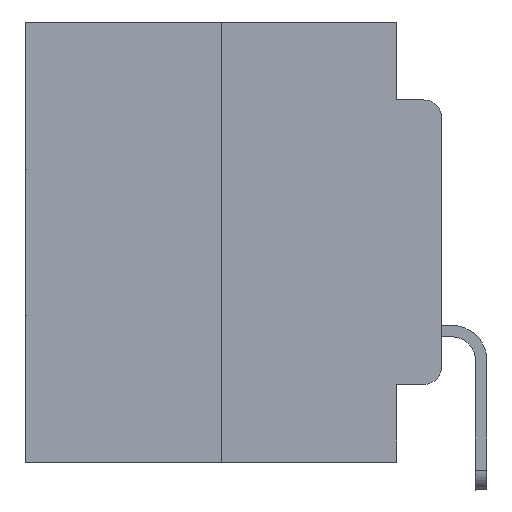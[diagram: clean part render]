
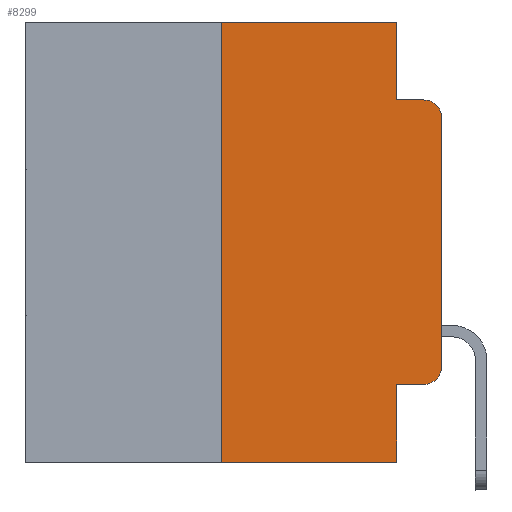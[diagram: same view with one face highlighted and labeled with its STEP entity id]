
A CAD part, left-side view. The second image highlights one B-rep face of the part: STEP entity #8299.
In plain terms, the highlighted planar face has unit normal (-1, 0, 0).
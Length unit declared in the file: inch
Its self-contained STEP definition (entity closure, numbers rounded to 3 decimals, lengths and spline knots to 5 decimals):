
#231 = EDGE_CURVE ( 'NONE', #22024, #13875, #4249, .T. ) ;
#243 = EDGE_CURVE ( 'NONE', #16934, #6753, #7136, .T. ) ;
#451 = CARTESIAN_POINT ( 'NONE',  ( 0., 0.051, 0. ) ) ;
#801 = ORIENTED_EDGE ( 'NONE', *, *, #7819, .T. ) ;
#1180 = AXIS2_PLACEMENT_3D ( 'NONE', #3368, #20275, #26350 ) ;
#1366 = EDGE_CURVE ( 'NONE', #1755, #2538, #14236, .T. ) ;
#1501 = EDGE_LOOP ( 'NONE', ( #801, #6724, #10126, #22751, #17772, #27119, #16622, #11106, #7341, #23350 ) ) ;
#1755 = VERTEX_POINT ( 'NONE', #24566 ) ;
#1921 = VERTEX_POINT ( 'NONE', #24707 ) ;
#2258 = LINE ( 'NONE', #17057, #8096 ) ;
#2538 = VERTEX_POINT ( 'NONE', #17056 ) ;
#3125 = CARTESIAN_POINT ( 'NONE',  ( 0., 0.02, -0.0885 ) ) ;
#3368 = CARTESIAN_POINT ( 'NONE',  ( 0., 0.473, 0. ) ) ;
#3680 = CARTESIAN_POINT ( 'NONE',  ( 0., 0.051, -0.4115 ) ) ;
#4249 = LINE ( 'NONE', #14787, #23830 ) ;
#4804 = LINE ( 'NONE', #21695, #24120 ) ;
#5696 = EDGE_CURVE ( 'NONE', #18847, #15049, #24532, .T. ) ;
#5939 = DIRECTION ( 'NONE',  ( -1., 0., 0. ) ) ;
#6724 = ORIENTED_EDGE ( 'NONE', *, *, #243, .T. ) ;
#6753 = VERTEX_POINT ( 'NONE', #3125 ) ;
#7136 = CIRCLE ( 'NONE', #12796, 0.02 ) ;
#7341 = ORIENTED_EDGE ( 'NONE', *, *, #8076, .T. ) ;
#7819 = EDGE_CURVE ( 'NONE', #15049, #16934, #9240, .T. ) ;
#7847 = EDGE_CURVE ( 'NONE', #1921, #22024, #4804, .T. ) ;
#7878 = CARTESIAN_POINT ( 'NONE',  ( 0., 0.02, -0.3915 ) ) ;
#7927 = CARTESIAN_POINT ( 'NONE',  ( 0., 0., -0.1085 ) ) ;
#8076 = EDGE_CURVE ( 'NONE', #1755, #18847, #10615, .T. ) ;
#8096 = VECTOR ( 'NONE', #25489, 39.37008 ) ;
#8299 = ADVANCED_FACE ( 'NONE', ( #9482 ), #19866, .F. ) ;
#8949 = EDGE_CURVE ( 'NONE', #13875, #24169, #19257, .T. ) ;
#9240 = LINE ( 'NONE', #15200, #13538 ) ;
#9482 = FACE_OUTER_BOUND ( 'NONE', #1501, .T. ) ;
#9534 = CARTESIAN_POINT ( 'NONE',  ( 0., 0.051, 0. ) ) ;
#10126 = ORIENTED_EDGE ( 'NONE', *, *, #25002, .F. ) ;
#10421 = AXIS2_PLACEMENT_3D ( 'NONE', #7878, #5939, #20496 ) ;
#10615 = LINE ( 'NONE', #3680, #26804 ) ;
#11106 = ORIENTED_EDGE ( 'NONE', *, *, #1366, .F. ) ;
#11527 = CARTESIAN_POINT ( 'NONE',  ( 0., 0.051, -0.0885 ) ) ;
#11593 = CARTESIAN_POINT ( 'NONE',  ( 0., 0.051, -0.0885 ) ) ;
#11717 = DIRECTION ( 'NONE',  ( 0., 0., 1. ) ) ;
#11862 = LINE ( 'NONE', #11593, #21523 ) ;
#12420 = DIRECTION ( 'NONE',  ( 0., -1., 0. ) ) ;
#12516 = CARTESIAN_POINT ( 'NONE',  ( 0., 0., -0.3915 ) ) ;
#12796 = AXIS2_PLACEMENT_3D ( 'NONE', #24731, #27213, #26945 ) ;
#13538 = VECTOR ( 'NONE', #15337, 39.37008 ) ;
#13875 = VERTEX_POINT ( 'NONE', #17110 ) ;
#14217 = DIRECTION ( 'NONE',  ( 0., -1., 0. ) ) ;
#14236 = LINE ( 'NONE', #9534, #20130 ) ;
#14787 = CARTESIAN_POINT ( 'NONE',  ( 0., 0.473, 0. ) ) ;
#15049 = VERTEX_POINT ( 'NONE', #12516 ) ;
#15200 = CARTESIAN_POINT ( 'NONE',  ( 0., 0., 0. ) ) ;
#15337 = DIRECTION ( 'NONE',  ( 0., 0., 1. ) ) ;
#16622 = ORIENTED_EDGE ( 'NONE', *, *, #19608, .T. ) ;
#16682 = VECTOR ( 'NONE', #25470, 39.37008 ) ;
#16703 = CARTESIAN_POINT ( 'NONE',  ( 0., 0.02, -0.4115 ) ) ;
#16934 = VERTEX_POINT ( 'NONE', #7927 ) ;
#17056 = CARTESIAN_POINT ( 'NONE',  ( 0., 0.051, -0.5 ) ) ;
#17057 = CARTESIAN_POINT ( 'NONE',  ( 0., 0.473, -0.5 ) ) ;
#17110 = CARTESIAN_POINT ( 'NONE',  ( 0., 0.051, 0. ) ) ;
#17772 = ORIENTED_EDGE ( 'NONE', *, *, #231, .F. ) ;
#18847 = VERTEX_POINT ( 'NONE', #16703 ) ;
#19257 = LINE ( 'NONE', #451, #16682 ) ;
#19608 = EDGE_CURVE ( 'NONE', #1921, #2538, #2258, .T. ) ;
#19866 = PLANE ( 'NONE',  #1180 ) ;
#20047 = DIRECTION ( 'NONE',  ( 0., -1., 0. ) ) ;
#20130 = VECTOR ( 'NONE', #26678, 39.37008 ) ;
#20275 = DIRECTION ( 'NONE',  ( 1., 0., 0. ) ) ;
#20496 = DIRECTION ( 'NONE',  ( 0., 0., -1. ) ) ;
#21523 = VECTOR ( 'NONE', #20047, 39.37008 ) ;
#21695 = CARTESIAN_POINT ( 'NONE',  ( 0., 0.25, 0. ) ) ;
#22024 = VERTEX_POINT ( 'NONE', #25775 ) ;
#22751 = ORIENTED_EDGE ( 'NONE', *, *, #8949, .F. ) ;
#23350 = ORIENTED_EDGE ( 'NONE', *, *, #5696, .T. ) ;
#23830 = VECTOR ( 'NONE', #12420, 39.37008 ) ;
#24120 = VECTOR ( 'NONE', #11717, 39.37008 ) ;
#24169 = VERTEX_POINT ( 'NONE', #11527 ) ;
#24532 = CIRCLE ( 'NONE', #10421, 0.02 ) ;
#24566 = CARTESIAN_POINT ( 'NONE',  ( 0., 0.051, -0.4115 ) ) ;
#24707 = CARTESIAN_POINT ( 'NONE',  ( 0., 0.25, -0.5 ) ) ;
#24731 = CARTESIAN_POINT ( 'NONE',  ( 0., 0.02, -0.1085 ) ) ;
#25002 = EDGE_CURVE ( 'NONE', #24169, #6753, #11862, .T. ) ;
#25470 = DIRECTION ( 'NONE',  ( 0., 0., -1. ) ) ;
#25489 = DIRECTION ( 'NONE',  ( 0., -1., 0. ) ) ;
#25775 = CARTESIAN_POINT ( 'NONE',  ( 0., 0.25, 0. ) ) ;
#26350 = DIRECTION ( 'NONE',  ( 0., 0., -1. ) ) ;
#26678 = DIRECTION ( 'NONE',  ( 0., 0., -1. ) ) ;
#26804 = VECTOR ( 'NONE', #14217, 39.37008 ) ;
#26945 = DIRECTION ( 'NONE',  ( 0., 0., -1. ) ) ;
#27119 = ORIENTED_EDGE ( 'NONE', *, *, #7847, .F. ) ;
#27213 = DIRECTION ( 'NONE',  ( -1., 0., 0. ) ) ;
